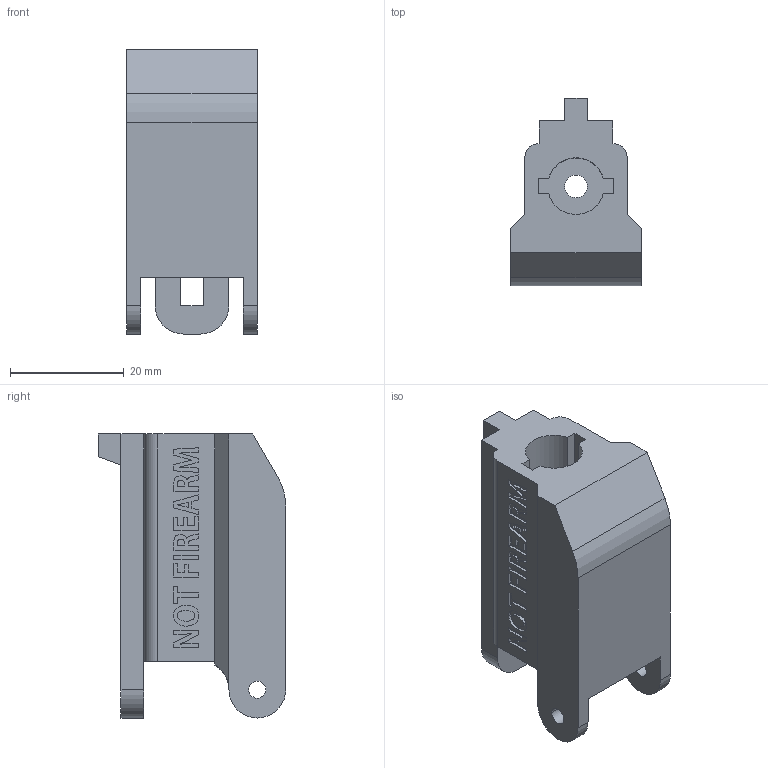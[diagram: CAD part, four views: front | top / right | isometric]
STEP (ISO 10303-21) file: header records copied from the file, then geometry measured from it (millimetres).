
FILE_DESCRIPTION (( 'STEP AP214' ), '1' );
FILE_NAME ('ParlorMod^CabooseParlor.STEP', '2014-10-07T00:03:07', ( 'WarFairy' ), ( '' ), 'SwSTEP 2.0', 'SolidWorks 2013', '' );
FILE_SCHEMA (( 'AUTOMOTIVE_DESIGN' ));
Length unit declared in the file: millimetre
Products named in the file (1): ParlorMod^CabooseParlor
Bounding box: 23 x 33 x 50 mm (x, y, z)
Volume: 18867.3 mm3; surface area: 7461.2 mm2
Topology: 1 solids, 1 shells, 261 faces, 700 edges, 464 vertices
Faces by surface type: plane 176, bspline 66, cylinder 19
Entity records: 11014 total; most frequent: CARTESIAN_POINT 4850, ORIENTED_EDGE 1400, DIRECTION 996, EDGE_CURVE 700, VECTOR 528, LINE 528, VERTEX_POINT 464, EDGE_LOOP 292
